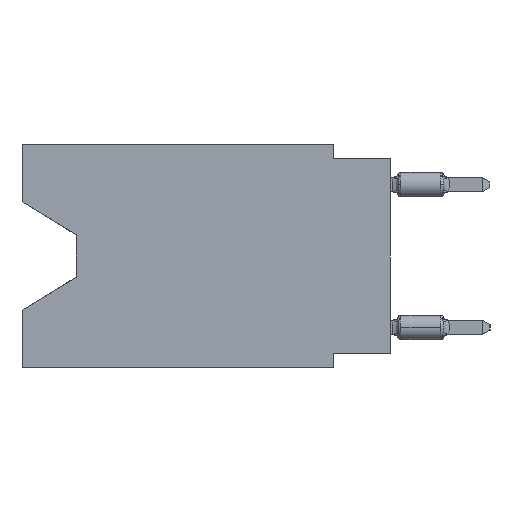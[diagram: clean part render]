
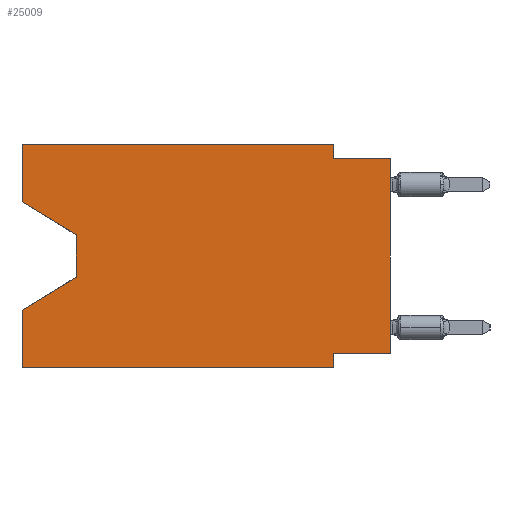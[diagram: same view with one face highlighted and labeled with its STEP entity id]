
A CAD part, left-side view. The second image highlights one B-rep face of the part: STEP entity #25009.
In plain terms, the highlighted planar face has unit normal (-1, 0, 0).
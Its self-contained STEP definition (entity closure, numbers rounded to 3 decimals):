
#172 = DIRECTION ( 'NONE',  ( 0., 1., 0. ) ) ;
#442 = DIRECTION ( 'NONE',  ( 0., 0., -1. ) ) ;
#662 = CARTESIAN_POINT ( 'NONE',  ( 0., 0., -0.635 ) ) ;
#751 = VERTEX_POINT ( 'NONE', #29956 ) ;
#916 = EDGE_CURVE ( 'NONE', #30080, #8987, #2894, .T. ) ;
#1479 = CARTESIAN_POINT ( 'NONE',  ( 0., 16.383, 0. ) ) ;
#1780 = CARTESIAN_POINT ( 'NONE',  ( 0., 16.383, 0. ) ) ;
#2246 = PLANE ( 'NONE',  #25773 ) ;
#2281 = DIRECTION ( 'NONE',  ( 0., 0., 1. ) ) ;
#2344 = VECTOR ( 'NONE', #6530, 1000. ) ;
#2353 = ORIENTED_EDGE ( 'NONE', *, *, #29271, .T. ) ;
#2894 = LINE ( 'NONE', #22334, #13369 ) ;
#2924 = CARTESIAN_POINT ( 'NONE',  ( 0., 13.97, -4.013 ) ) ;
#3078 = VERTEX_POINT ( 'NONE', #26743 ) ;
#3607 = LINE ( 'NONE', #15786, #23493 ) ;
#3677 = VECTOR ( 'NONE', #20644, 1000. ) ;
#3817 = ORIENTED_EDGE ( 'NONE', *, *, #5226, .F. ) ;
#4553 = CARTESIAN_POINT ( 'NONE',  ( 0., 2.54, 0. ) ) ;
#5226 = EDGE_CURVE ( 'NONE', #751, #27282, #13555, .T. ) ;
#5280 = VERTEX_POINT ( 'NONE', #11810 ) ;
#5463 = LINE ( 'NONE', #2924, #29287 ) ;
#6530 = DIRECTION ( 'NONE',  ( 0., -1., 0. ) ) ;
#6754 = VECTOR ( 'NONE', #2281, 1000. ) ;
#7032 = CARTESIAN_POINT ( 'NONE',  ( 0., 0., 0. ) ) ;
#7366 = VERTEX_POINT ( 'NONE', #27514 ) ;
#7688 = CARTESIAN_POINT ( 'NONE',  ( 0., 16.383, 0. ) ) ;
#8779 = DIRECTION ( 'NONE',  ( 0., 0., 1. ) ) ;
#8987 = VERTEX_POINT ( 'NONE', #19624 ) ;
#9952 = VERTEX_POINT ( 'NONE', #17017 ) ;
#9961 = ORIENTED_EDGE ( 'NONE', *, *, #19436, .F. ) ;
#10179 = DIRECTION ( 'NONE',  ( 0., -0.855, -0.519 ) ) ;
#10351 = DIRECTION ( 'NONE',  ( 0., 0., -1. ) ) ;
#11242 = CARTESIAN_POINT ( 'NONE',  ( 0., 16.383, -2.546 ) ) ;
#11648 = ORIENTED_EDGE ( 'NONE', *, *, #19669, .T. ) ;
#11810 = CARTESIAN_POINT ( 'NONE',  ( 0., 2.54, -9.271 ) ) ;
#11901 = DIRECTION ( 'NONE',  ( 1., 0., 0. ) ) ;
#12147 = CARTESIAN_POINT ( 'NONE',  ( 0., 2.54, -9.906 ) ) ;
#12266 = VERTEX_POINT ( 'NONE', #16129 ) ;
#13369 = VECTOR ( 'NONE', #10179, 1000. ) ;
#13372 = CARTESIAN_POINT ( 'NONE',  ( 0., 2.54, 0. ) ) ;
#13555 = LINE ( 'NONE', #23178, #22585 ) ;
#13896 = VECTOR ( 'NONE', #172, 1000. ) ;
#14099 = CARTESIAN_POINT ( 'NONE',  ( 0., 2.54, -9.906 ) ) ;
#14243 = CARTESIAN_POINT ( 'NONE',  ( 0., 0., -9.271 ) ) ;
#14597 = CARTESIAN_POINT ( 'NONE',  ( 0., 16.383, 0. ) ) ;
#14759 = DIRECTION ( 'NONE',  ( 0., -1., 0. ) ) ;
#15374 = EDGE_CURVE ( 'NONE', #8987, #12266, #5463, .T. ) ;
#15408 = ORIENTED_EDGE ( 'NONE', *, *, #26585, .F. ) ;
#15554 = ORIENTED_EDGE ( 'NONE', *, *, #27327, .T. ) ;
#15786 = CARTESIAN_POINT ( 'NONE',  ( 0., 13.97, -5.893 ) ) ;
#16106 = VERTEX_POINT ( 'NONE', #14099 ) ;
#16129 = CARTESIAN_POINT ( 'NONE',  ( 0., 13.97, -5.893 ) ) ;
#16698 = EDGE_LOOP ( 'NONE', ( #21914, #28264, #11648, #23438, #15554, #23676, #9961, #2353, #3817, #17404, #28220, #15408 ) ) ;
#16812 = VECTOR ( 'NONE', #27546, 1000. ) ;
#17017 = CARTESIAN_POINT ( 'NONE',  ( 0., 16.383, -7.36 ) ) ;
#17404 = ORIENTED_EDGE ( 'NONE', *, *, #26593, .F. ) ;
#19436 = EDGE_CURVE ( 'NONE', #7366, #5280, #21808, .T. ) ;
#19578 = VECTOR ( 'NONE', #442, 1000. ) ;
#19624 = CARTESIAN_POINT ( 'NONE',  ( 0., 13.97, -4.013 ) ) ;
#19669 = EDGE_CURVE ( 'NONE', #12266, #9952, #3607, .T. ) ;
#19743 = VERTEX_POINT ( 'NONE', #30761 ) ;
#20644 = DIRECTION ( 'NONE',  ( 0., 0., -1. ) ) ;
#21696 = DIRECTION ( 'NONE',  ( 0., 0., -1. ) ) ;
#21808 = LINE ( 'NONE', #14243, #13896 ) ;
#21914 = ORIENTED_EDGE ( 'NONE', *, *, #916, .T. ) ;
#22163 = CARTESIAN_POINT ( 'NONE',  ( 0., 16.383, -9.906 ) ) ;
#22334 = CARTESIAN_POINT ( 'NONE',  ( 0., 16.383, -2.546 ) ) ;
#22585 = VECTOR ( 'NONE', #29813, 1000. ) ;
#23123 = LINE ( 'NONE', #1479, #16812 ) ;
#23154 = LINE ( 'NONE', #13372, #3677 ) ;
#23178 = CARTESIAN_POINT ( 'NONE',  ( 0., 0., -0.635 ) ) ;
#23356 = VECTOR ( 'NONE', #8779, 1000. ) ;
#23438 = ORIENTED_EDGE ( 'NONE', *, *, #28286, .F. ) ;
#23493 = VECTOR ( 'NONE', #25408, 1000. ) ;
#23676 = ORIENTED_EDGE ( 'NONE', *, *, #24215, .F. ) ;
#24046 = VERTEX_POINT ( 'NONE', #4553 ) ;
#24215 = EDGE_CURVE ( 'NONE', #5280, #16106, #26967, .T. ) ;
#24522 = LINE ( 'NONE', #22163, #30445 ) ;
#25009 = ADVANCED_FACE ( 'NONE', ( #26577 ), #2246, .F. ) ;
#25408 = DIRECTION ( 'NONE',  ( 0., 0.855, -0.519 ) ) ;
#25648 = LINE ( 'NONE', #1780, #2344 ) ;
#25773 = AXIS2_PLACEMENT_3D ( 'NONE', #14597, #11901, #21696 ) ;
#26577 = FACE_OUTER_BOUND ( 'NONE', #16698, .T. ) ;
#26585 = EDGE_CURVE ( 'NONE', #30080, #3078, #29344, .T. ) ;
#26593 = EDGE_CURVE ( 'NONE', #24046, #751, #23154, .T. ) ;
#26743 = CARTESIAN_POINT ( 'NONE',  ( 0., 16.383, 0. ) ) ;
#26967 = LINE ( 'NONE', #12147, #19578 ) ;
#27282 = VERTEX_POINT ( 'NONE', #662 ) ;
#27327 = EDGE_CURVE ( 'NONE', #19743, #16106, #24522, .T. ) ;
#27514 = CARTESIAN_POINT ( 'NONE',  ( 0., 0., -9.271 ) ) ;
#27546 = DIRECTION ( 'NONE',  ( 0., 0., 1. ) ) ;
#28220 = ORIENTED_EDGE ( 'NONE', *, *, #30998, .F. ) ;
#28264 = ORIENTED_EDGE ( 'NONE', *, *, #15374, .T. ) ;
#28286 = EDGE_CURVE ( 'NONE', #19743, #9952, #23123, .T. ) ;
#29271 = EDGE_CURVE ( 'NONE', #7366, #27282, #31031, .T. ) ;
#29287 = VECTOR ( 'NONE', #10351, 1000. ) ;
#29344 = LINE ( 'NONE', #7688, #23356 ) ;
#29813 = DIRECTION ( 'NONE',  ( 0., -1., 0. ) ) ;
#29956 = CARTESIAN_POINT ( 'NONE',  ( 0., 2.54, -0.635 ) ) ;
#30080 = VERTEX_POINT ( 'NONE', #11242 ) ;
#30445 = VECTOR ( 'NONE', #14759, 1000. ) ;
#30761 = CARTESIAN_POINT ( 'NONE',  ( 0., 16.383, -9.906 ) ) ;
#30998 = EDGE_CURVE ( 'NONE', #3078, #24046, #25648, .T. ) ;
#31031 = LINE ( 'NONE', #7032, #6754 ) ;
